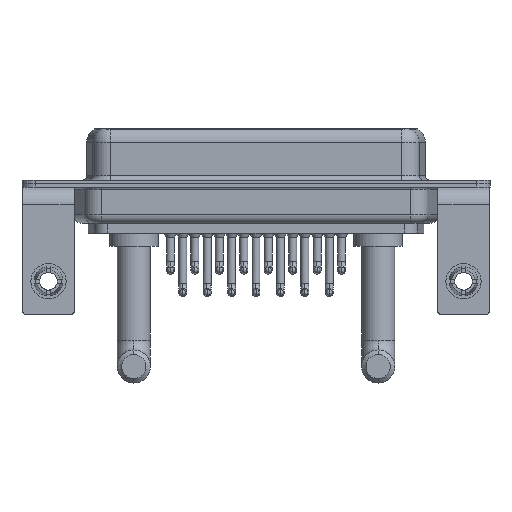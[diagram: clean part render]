
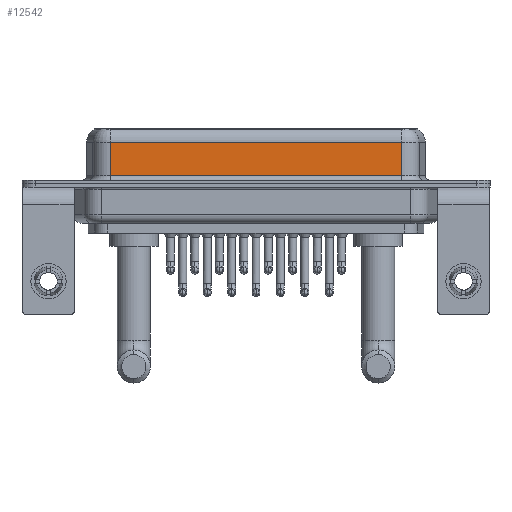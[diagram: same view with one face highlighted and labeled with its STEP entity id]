
A CAD part, front view. The second image highlights one B-rep face of the part: STEP entity #12542.
In plain terms, the highlighted planar face has unit normal (0, -1, 0).
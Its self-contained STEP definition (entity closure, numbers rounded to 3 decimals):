
#122 = EDGE_LOOP ( 'NONE', ( #12746, #21482, #15560, #18834 ) ) ;
#387 = LINE ( 'NONE', #21989, #21660 ) ;
#1849 = CARTESIAN_POINT ( 'NONE',  ( 40.037, -3.95, 0.9 ) ) ;
#3731 = DIRECTION ( 'NONE',  ( 0., 0., -1. ) ) ;
#3785 = DIRECTION ( 'NONE',  ( 0., 0., -1. ) ) ;
#5107 = VECTOR ( 'NONE', #15113, 1000. ) ;
#6580 = CARTESIAN_POINT ( 'NONE',  ( 40.037, -3.95, 0.9 ) ) ;
#6763 = VERTEX_POINT ( 'NONE', #15578 ) ;
#7244 = DIRECTION ( 'NONE',  ( 1., 0., 0. ) ) ;
#7748 = VECTOR ( 'NONE', #3731, 1000. ) ;
#12542 = ADVANCED_FACE ( 'NONE', ( #15215 ), #22347, .F. ) ;
#12580 = VERTEX_POINT ( 'NONE', #6580 ) ;
#12706 = LINE ( 'NONE', #18075, #7748 ) ;
#12746 = ORIENTED_EDGE ( 'NONE', *, *, #17705, .F. ) ;
#12891 = CARTESIAN_POINT ( 'NONE',  ( 40.037, -3.95, 6.4 ) ) ;
#13098 = VERTEX_POINT ( 'NONE', #19024 ) ;
#14999 = LINE ( 'NONE', #22357, #5107 ) ;
#15113 = DIRECTION ( 'NONE',  ( -1., 0., 0. ) ) ;
#15215 = FACE_OUTER_BOUND ( 'NONE', #122, .T. ) ;
#15560 = ORIENTED_EDGE ( 'NONE', *, *, #21208, .T. ) ;
#15578 = CARTESIAN_POINT ( 'NONE',  ( 40.037, -3.95, 4.65 ) ) ;
#17347 = AXIS2_PLACEMENT_3D ( 'NONE', #12891, #20015, #20128 ) ;
#17705 = EDGE_CURVE ( 'NONE', #6763, #12580, #12706, .T. ) ;
#17946 = LINE ( 'NONE', #1849, #22405 ) ;
#18075 = CARTESIAN_POINT ( 'NONE',  ( 40.037, -3.95, 6.4 ) ) ;
#18199 = EDGE_CURVE ( 'NONE', #6763, #13098, #14999, .T. ) ;
#18834 = ORIENTED_EDGE ( 'NONE', *, *, #18882, .T. ) ;
#18882 = EDGE_CURVE ( 'NONE', #20197, #12580, #17946, .T. ) ;
#19024 = CARTESIAN_POINT ( 'NONE',  ( 7.013, -3.95, 4.65 ) ) ;
#19152 = CARTESIAN_POINT ( 'NONE',  ( 7.013, -3.95, 0.9 ) ) ;
#20015 = DIRECTION ( 'NONE',  ( 0., 1., 0. ) ) ;
#20128 = DIRECTION ( 'NONE',  ( 0., 0., 1. ) ) ;
#20197 = VERTEX_POINT ( 'NONE', #19152 ) ;
#21208 = EDGE_CURVE ( 'NONE', #13098, #20197, #387, .T. ) ;
#21482 = ORIENTED_EDGE ( 'NONE', *, *, #18199, .T. ) ;
#21660 = VECTOR ( 'NONE', #3785, 1000. ) ;
#21989 = CARTESIAN_POINT ( 'NONE',  ( 7.013, -3.95, 6.4 ) ) ;
#22347 = PLANE ( 'NONE',  #17347 ) ;
#22357 = CARTESIAN_POINT ( 'NONE',  ( 40.037, -3.95, 4.65 ) ) ;
#22405 = VECTOR ( 'NONE', #7244, 1000. ) ;
